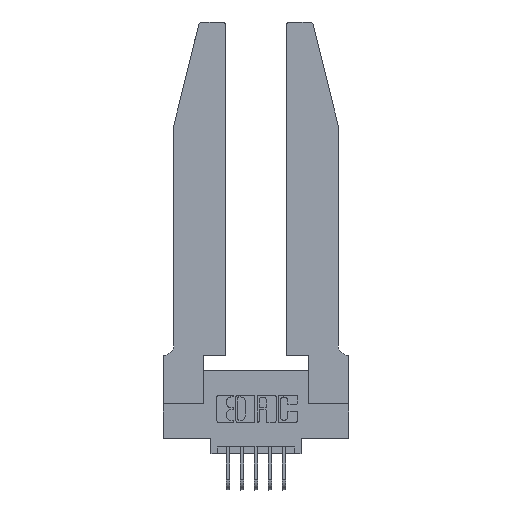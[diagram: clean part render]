
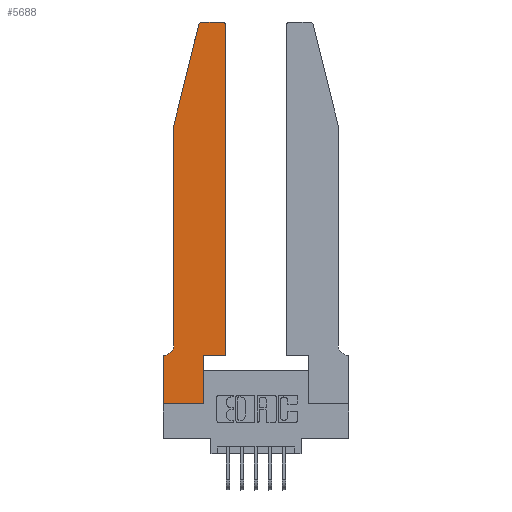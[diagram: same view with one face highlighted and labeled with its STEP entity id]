
A CAD part, top view. The second image highlights one B-rep face of the part: STEP entity #5688.
In plain terms, the highlighted planar face has unit normal (0, 0, 1).
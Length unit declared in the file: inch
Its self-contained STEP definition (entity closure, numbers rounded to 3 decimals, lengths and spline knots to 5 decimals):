
#166 = DIRECTION ( 'NONE',  ( 0., 0., -1. ) ) ;
#220 = DIRECTION ( 'NONE',  ( 1., 0., 0. ) ) ;
#485 = CIRCLE ( 'NONE', #2434, 0.03 ) ;
#593 = CIRCLE ( 'NONE', #13465, 0.03 ) ;
#730 = LINE ( 'NONE', #9575, #3294 ) ;
#780 = CARTESIAN_POINT ( 'NONE',  ( 0.0055, 0.35, 0.37 ) ) ;
#1038 = EDGE_CURVE ( 'NONE', #10918, #11756, #4956, .T. ) ;
#1060 = VERTEX_POINT ( 'NONE', #3747 ) ;
#1132 = EDGE_CURVE ( 'NONE', #11756, #7138, #4606, .T. ) ;
#1537 = DIRECTION ( 'NONE',  ( 0., 0., 1. ) ) ;
#1664 = VERTEX_POINT ( 'NONE', #4547 ) ;
#1831 = CARTESIAN_POINT ( 'NONE',  ( 0.0755, 2., 0.37 ) ) ;
#2132 = VECTOR ( 'NONE', #8839, 39.37008 ) ;
#2173 = DIRECTION ( 'NONE',  ( -1., 0., 0. ) ) ;
#2434 = AXIS2_PLACEMENT_3D ( 'NONE', #7913, #1537, #8971 ) ;
#2800 = ORIENTED_EDGE ( 'NONE', *, *, #1132, .T. ) ;
#2919 = DIRECTION ( 'NONE',  ( -0.239, -0.971, 0. ) ) ;
#3294 = VECTOR ( 'NONE', #2173, 39.37008 ) ;
#3335 = CARTESIAN_POINT ( 'NONE',  ( 0.4505, 2.72, 0.37 ) ) ;
#3747 = CARTESIAN_POINT ( 'NONE',  ( 0.25487, 2.72718, 0.37 ) ) ;
#3783 = CARTESIAN_POINT ( 'NONE',  ( 0.0755, 0.42, 0.37 ) ) ;
#3819 = LINE ( 'NONE', #9175, #6290 ) ;
#3833 = CARTESIAN_POINT ( 'NONE',  ( 0., 0.35, 0.37 ) ) ;
#4006 = DIRECTION ( 'NONE',  ( 1., 0., 0. ) ) ;
#4109 = EDGE_CURVE ( 'NONE', #9399, #6943, #10106, .T. ) ;
#4119 = CARTESIAN_POINT ( 'NONE',  ( 0.2865, 0.35, 0.37 ) ) ;
#4180 = CARTESIAN_POINT ( 'NONE',  ( 0., 0., 0.37 ) ) ;
#4211 = EDGE_CURVE ( 'NONE', #7138, #9399, #6025, .T. ) ;
#4547 = CARTESIAN_POINT ( 'NONE',  ( 0.0755, 2., 0.37 ) ) ;
#4606 = LINE ( 'NONE', #4180, #11997 ) ;
#4696 = LINE ( 'NONE', #1831, #5370 ) ;
#4956 = LINE ( 'NONE', #6860, #10507 ) ;
#5002 = DIRECTION ( 'NONE',  ( 0., 1., 0. ) ) ;
#5031 = ORIENTED_EDGE ( 'NONE', *, *, #5114, .T. ) ;
#5114 = EDGE_CURVE ( 'NONE', #1060, #1664, #4696, .T. ) ;
#5339 = LINE ( 'NONE', #11931, #2132 ) ;
#5370 = VECTOR ( 'NONE', #2919, 39.37008 ) ;
#5688 = ADVANCED_FACE ( 'NONE', ( #8620 ), #12265, .T. ) ;
#5961 = EDGE_CURVE ( 'NONE', #6887, #10918, #10404, .T. ) ;
#5992 = CARTESIAN_POINT ( 'NONE',  ( 0., 0.35, 0.37 ) ) ;
#6025 = LINE ( 'NONE', #4119, #11272 ) ;
#6290 = VECTOR ( 'NONE', #5002, 39.37008 ) ;
#6302 = ORIENTED_EDGE ( 'NONE', *, *, #10087, .T. ) ;
#6309 = ORIENTED_EDGE ( 'NONE', *, *, #13067, .T. ) ;
#6518 = VERTEX_POINT ( 'NONE', #7580 ) ;
#6634 = CARTESIAN_POINT ( 'NONE',  ( 0.0055, 0.42, 0.37 ) ) ;
#6686 = DIRECTION ( 'NONE',  ( 0., 0., 1. ) ) ;
#6860 = CARTESIAN_POINT ( 'NONE',  ( 0., 0., 0.37 ) ) ;
#6887 = VERTEX_POINT ( 'NONE', #780 ) ;
#6943 = VERTEX_POINT ( 'NONE', #7260 ) ;
#6952 = DIRECTION ( 'NONE',  ( 0., -1., 0. ) ) ;
#7062 = DIRECTION ( 'NONE',  ( 1., 0., 0. ) ) ;
#7070 = EDGE_CURVE ( 'NONE', #7394, #6518, #730, .T. ) ;
#7138 = VERTEX_POINT ( 'NONE', #9673 ) ;
#7260 = CARTESIAN_POINT ( 'NONE',  ( 0.4505, 0.35, 0.37 ) ) ;
#7348 = CARTESIAN_POINT ( 'NONE',  ( 0., 0., 0.37 ) ) ;
#7394 = VERTEX_POINT ( 'NONE', #10242 ) ;
#7580 = CARTESIAN_POINT ( 'NONE',  ( 0.284, 2.75, 0.37 ) ) ;
#7661 = VERTEX_POINT ( 'NONE', #3335 ) ;
#7669 = DIRECTION ( 'NONE',  ( -1., 0., 0. ) ) ;
#7849 = EDGE_CURVE ( 'NONE', #6518, #1060, #485, .T. ) ;
#7913 = CARTESIAN_POINT ( 'NONE',  ( 0.284, 2.72, 0.37 ) ) ;
#8227 = ORIENTED_EDGE ( 'NONE', *, *, #10963, .T. ) ;
#8422 = CARTESIAN_POINT ( 'NONE',  ( 0.2865, 0.35, 0.37 ) ) ;
#8546 = AXIS2_PLACEMENT_3D ( 'NONE', #6634, #166, #7669 ) ;
#8620 = FACE_OUTER_BOUND ( 'NONE', #11123, .T. ) ;
#8839 = DIRECTION ( 'NONE',  ( 0., -1., 0. ) ) ;
#8971 = DIRECTION ( 'NONE',  ( 1., 0., 0. ) ) ;
#9175 = CARTESIAN_POINT ( 'NONE',  ( 0.4505, 0.35, 0.37 ) ) ;
#9399 = VERTEX_POINT ( 'NONE', #8422 ) ;
#9575 = CARTESIAN_POINT ( 'NONE',  ( 0.2605, 2.75, 0.37 ) ) ;
#9673 = CARTESIAN_POINT ( 'NONE',  ( 0.2865, 0., 0.37 ) ) ;
#9839 = CARTESIAN_POINT ( 'NONE',  ( 0.0755, 0.35, 0.37 ) ) ;
#9902 = ORIENTED_EDGE ( 'NONE', *, *, #10045, .T. ) ;
#10045 = EDGE_CURVE ( 'NONE', #7661, #7394, #593, .T. ) ;
#10087 = EDGE_CURVE ( 'NONE', #1664, #10863, #5339, .T. ) ;
#10106 = LINE ( 'NONE', #12392, #12569 ) ;
#10242 = CARTESIAN_POINT ( 'NONE',  ( 0.4205, 2.75, 0.37 ) ) ;
#10269 = DIRECTION ( 'NONE',  ( 1., 0., 0. ) ) ;
#10404 = LINE ( 'NONE', #9839, #13656 ) ;
#10507 = VECTOR ( 'NONE', #6952, 39.37008 ) ;
#10809 = ORIENTED_EDGE ( 'NONE', *, *, #1038, .T. ) ;
#10863 = VERTEX_POINT ( 'NONE', #3783 ) ;
#10918 = VERTEX_POINT ( 'NONE', #3833 ) ;
#10963 = EDGE_CURVE ( 'NONE', #6943, #7661, #3819, .T. ) ;
#11123 = EDGE_LOOP ( 'NONE', ( #11782, #11202, #5031, #6302, #6309, #11607, #10809, #2800, #12208, #12411, #8227, #9902 ) ) ;
#11202 = ORIENTED_EDGE ( 'NONE', *, *, #7849, .T. ) ;
#11272 = VECTOR ( 'NONE', #11488, 39.37008 ) ;
#11488 = DIRECTION ( 'NONE',  ( 0., 1., 0. ) ) ;
#11607 = ORIENTED_EDGE ( 'NONE', *, *, #5961, .T. ) ;
#11756 = VERTEX_POINT ( 'NONE', #7348 ) ;
#11782 = ORIENTED_EDGE ( 'NONE', *, *, #7070, .T. ) ;
#11931 = CARTESIAN_POINT ( 'NONE',  ( 0.0755, 2., 0.37 ) ) ;
#11950 = DIRECTION ( 'NONE',  ( -1., 0., 0. ) ) ;
#11997 = VECTOR ( 'NONE', #4006, 39.37008 ) ;
#12208 = ORIENTED_EDGE ( 'NONE', *, *, #4211, .T. ) ;
#12265 = PLANE ( 'NONE',  #13429 ) ;
#12392 = CARTESIAN_POINT ( 'NONE',  ( 0.4505, 0.35, 0.37 ) ) ;
#12411 = ORIENTED_EDGE ( 'NONE', *, *, #4109, .T. ) ;
#12569 = VECTOR ( 'NONE', #10269, 39.37008 ) ;
#12929 = CARTESIAN_POINT ( 'NONE',  ( 0.4205, 2.72, 0.37 ) ) ;
#13067 = EDGE_CURVE ( 'NONE', #10863, #6887, #13438, .T. ) ;
#13290 = DIRECTION ( 'NONE',  ( 0., 0., 1. ) ) ;
#13429 = AXIS2_PLACEMENT_3D ( 'NONE', #5992, #13290, #7062 ) ;
#13438 = CIRCLE ( 'NONE', #8546, 0.07 ) ;
#13465 = AXIS2_PLACEMENT_3D ( 'NONE', #12929, #6686, #220 ) ;
#13656 = VECTOR ( 'NONE', #11950, 39.37008 ) ;
